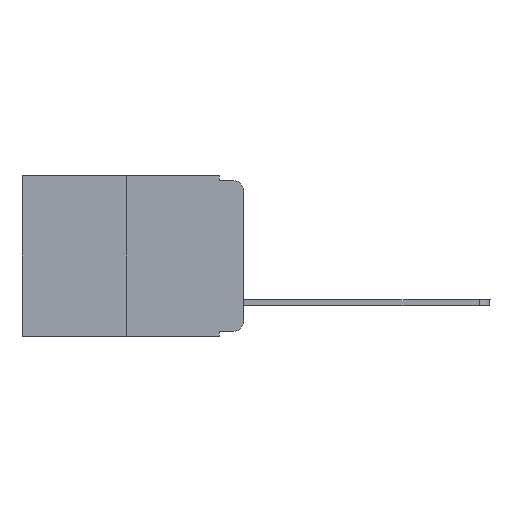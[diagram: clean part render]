
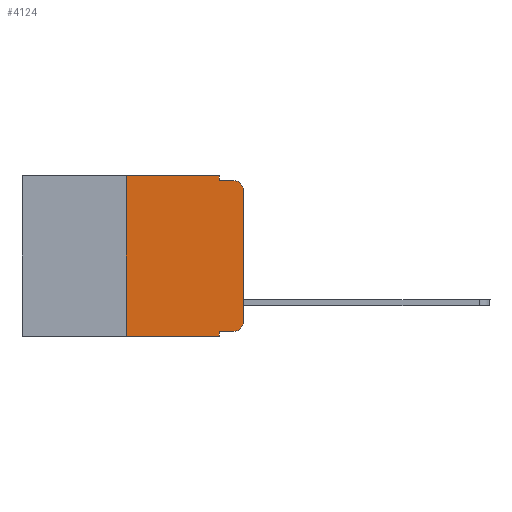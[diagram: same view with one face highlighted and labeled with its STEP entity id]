
A CAD part, left-side view. The second image highlights one B-rep face of the part: STEP entity #4124.
In plain terms, the highlighted planar face has unit normal (-1, 0, 0).
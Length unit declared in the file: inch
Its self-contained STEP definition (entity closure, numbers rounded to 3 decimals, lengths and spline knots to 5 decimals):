
#188 = CARTESIAN_POINT ( 'NONE',  ( 0., 0.051, -0.333 ) ) ;
#191 = CARTESIAN_POINT ( 'NONE',  ( 0., 0.473, 0. ) ) ;
#391 = VECTOR ( 'NONE', #13929, 39.37008 ) ;
#523 = EDGE_CURVE ( 'NONE', #12722, #14645, #2433, .T. ) ;
#609 = ORIENTED_EDGE ( 'NONE', *, *, #11654, .T. ) ;
#1378 = LINE ( 'NONE', #188, #7706 ) ;
#1513 = VECTOR ( 'NONE', #4745, 39.37008 ) ;
#1540 = DIRECTION ( 'NONE',  ( 0., 0., -1. ) ) ;
#1589 = CARTESIAN_POINT ( 'NONE',  ( 0., 0.25, 0. ) ) ;
#1885 = CARTESIAN_POINT ( 'NONE',  ( 0., 0.051, 0. ) ) ;
#2061 = LINE ( 'NONE', #4326, #11619 ) ;
#2253 = ORIENTED_EDGE ( 'NONE', *, *, #16123, .F. ) ;
#2433 = CIRCLE ( 'NONE', #3259, 0.02 ) ;
#2586 = VERTEX_POINT ( 'NONE', #12655 ) ;
#2613 = VERTEX_POINT ( 'NONE', #2933 ) ;
#2822 = EDGE_LOOP ( 'NONE', ( #6331, #609, #2930, #5200, #11646, #9759, #9044, #2253, #6408, #6726 ) ) ;
#2831 = VERTEX_POINT ( 'NONE', #16024 ) ;
#2930 = ORIENTED_EDGE ( 'NONE', *, *, #15070, .F. ) ;
#2933 = CARTESIAN_POINT ( 'NONE',  ( 0., 0.02, -0.01 ) ) ;
#3259 = AXIS2_PLACEMENT_3D ( 'NONE', #16410, #4919, #1540 ) ;
#3643 = DIRECTION ( 'NONE',  ( 0., -1., 0. ) ) ;
#3963 = CARTESIAN_POINT ( 'NONE',  ( 0., 0.051, -0.01 ) ) ;
#4054 = CARTESIAN_POINT ( 'NONE',  ( 0., 0., -0.313 ) ) ;
#4124 = ADVANCED_FACE ( 'NONE', ( #12852 ), #5401, .F. ) ;
#4326 = CARTESIAN_POINT ( 'NONE',  ( 0., 0.051, 0. ) ) ;
#4379 = DIRECTION ( 'NONE',  ( -1., 0., 0. ) ) ;
#4727 = VECTOR ( 'NONE', #3643, 39.37008 ) ;
#4745 = DIRECTION ( 'NONE',  ( 0., 0., 1. ) ) ;
#4813 = LINE ( 'NONE', #9921, #4727 ) ;
#4919 = DIRECTION ( 'NONE',  ( -1., 0., 0. ) ) ;
#5200 = ORIENTED_EDGE ( 'NONE', *, *, #16261, .F. ) ;
#5273 = CARTESIAN_POINT ( 'NONE',  ( 0., 0.051, -0.343 ) ) ;
#5401 = PLANE ( 'NONE',  #6969 ) ;
#5446 = VERTEX_POINT ( 'NONE', #9172 ) ;
#6137 = CARTESIAN_POINT ( 'NONE',  ( 0., 0.051, -0.333 ) ) ;
#6168 = EDGE_CURVE ( 'NONE', #2831, #9923, #9901, .T. ) ;
#6185 = VERTEX_POINT ( 'NONE', #6137 ) ;
#6331 = ORIENTED_EDGE ( 'NONE', *, *, #8968, .T. ) ;
#6408 = ORIENTED_EDGE ( 'NONE', *, *, #7410, .T. ) ;
#6457 = CIRCLE ( 'NONE', #11273, 0.02 ) ;
#6726 = ORIENTED_EDGE ( 'NONE', *, *, #523, .T. ) ;
#6969 = AXIS2_PLACEMENT_3D ( 'NONE', #191, #9169, #7921 ) ;
#6996 = EDGE_CURVE ( 'NONE', #5446, #14183, #4813, .T. ) ;
#7410 = EDGE_CURVE ( 'NONE', #6185, #12722, #1378, .T. ) ;
#7706 = VECTOR ( 'NONE', #11605, 39.37008 ) ;
#7921 = DIRECTION ( 'NONE',  ( 0., 0., -1. ) ) ;
#7978 = DIRECTION ( 'NONE',  ( 0., 0., 1. ) ) ;
#8198 = CARTESIAN_POINT ( 'NONE',  ( 0., 0.02, -0.333 ) ) ;
#8270 = LINE ( 'NONE', #1885, #13212 ) ;
#8814 = CARTESIAN_POINT ( 'NONE',  ( 0., 0.473, -0.343 ) ) ;
#8968 = EDGE_CURVE ( 'NONE', #14645, #2586, #11113, .T. ) ;
#9044 = ORIENTED_EDGE ( 'NONE', *, *, #6168, .T. ) ;
#9069 = DIRECTION ( 'NONE',  ( 0., -1., 0. ) ) ;
#9144 = EDGE_CURVE ( 'NONE', #2831, #5446, #10645, .T. ) ;
#9169 = DIRECTION ( 'NONE',  ( 1., 0., 0. ) ) ;
#9172 = CARTESIAN_POINT ( 'NONE',  ( 0., 0.25, 0. ) ) ;
#9295 = VECTOR ( 'NONE', #7978, 39.37008 ) ;
#9335 = DIRECTION ( 'NONE',  ( 0., 0., -1. ) ) ;
#9696 = DIRECTION ( 'NONE',  ( 0., 0., -1. ) ) ;
#9759 = ORIENTED_EDGE ( 'NONE', *, *, #9144, .F. ) ;
#9901 = LINE ( 'NONE', #8814, #391 ) ;
#9921 = CARTESIAN_POINT ( 'NONE',  ( 0., 0.473, 0. ) ) ;
#9923 = VERTEX_POINT ( 'NONE', #5273 ) ;
#10290 = CARTESIAN_POINT ( 'NONE',  ( 0., 0.051, 0. ) ) ;
#10335 = LINE ( 'NONE', #3963, #15637 ) ;
#10645 = LINE ( 'NONE', #1589, #9295 ) ;
#11113 = LINE ( 'NONE', #16236, #1513 ) ;
#11273 = AXIS2_PLACEMENT_3D ( 'NONE', #11833, #4379, #9335 ) ;
#11605 = DIRECTION ( 'NONE',  ( 0., -1., 0. ) ) ;
#11619 = VECTOR ( 'NONE', #9696, 39.37008 ) ;
#11646 = ORIENTED_EDGE ( 'NONE', *, *, #6996, .F. ) ;
#11654 = EDGE_CURVE ( 'NONE', #2586, #2613, #6457, .T. ) ;
#11833 = CARTESIAN_POINT ( 'NONE',  ( 0., 0.02, -0.03 ) ) ;
#12114 = DIRECTION ( 'NONE',  ( 0., 0., -1. ) ) ;
#12655 = CARTESIAN_POINT ( 'NONE',  ( 0., 0., -0.03 ) ) ;
#12722 = VERTEX_POINT ( 'NONE', #8198 ) ;
#12852 = FACE_OUTER_BOUND ( 'NONE', #2822, .T. ) ;
#13212 = VECTOR ( 'NONE', #12114, 39.37008 ) ;
#13929 = DIRECTION ( 'NONE',  ( 0., -1., 0. ) ) ;
#14183 = VERTEX_POINT ( 'NONE', #10290 ) ;
#14508 = VERTEX_POINT ( 'NONE', #15063 ) ;
#14645 = VERTEX_POINT ( 'NONE', #4054 ) ;
#15063 = CARTESIAN_POINT ( 'NONE',  ( 0., 0.051, -0.01 ) ) ;
#15070 = EDGE_CURVE ( 'NONE', #14508, #2613, #10335, .T. ) ;
#15637 = VECTOR ( 'NONE', #9069, 39.37008 ) ;
#16024 = CARTESIAN_POINT ( 'NONE',  ( 0., 0.25, -0.343 ) ) ;
#16123 = EDGE_CURVE ( 'NONE', #6185, #9923, #2061, .T. ) ;
#16236 = CARTESIAN_POINT ( 'NONE',  ( 0., 0., 0. ) ) ;
#16261 = EDGE_CURVE ( 'NONE', #14183, #14508, #8270, .T. ) ;
#16410 = CARTESIAN_POINT ( 'NONE',  ( 0., 0.02, -0.313 ) ) ;
